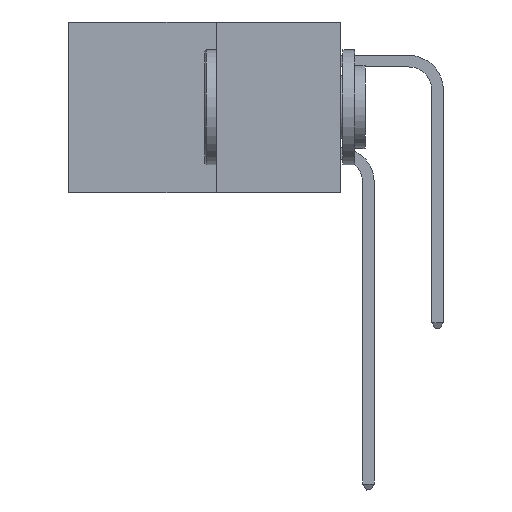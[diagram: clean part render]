
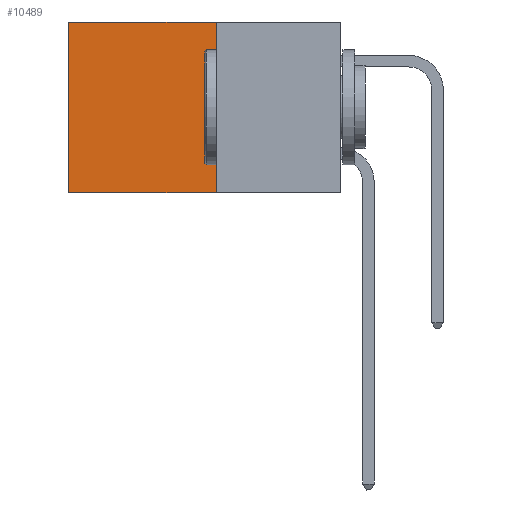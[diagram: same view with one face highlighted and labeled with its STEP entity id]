
A CAD part, left-side view. The second image highlights one B-rep face of the part: STEP entity #10489.
In plain terms, the highlighted planar face has unit normal (-1, 0, 0).
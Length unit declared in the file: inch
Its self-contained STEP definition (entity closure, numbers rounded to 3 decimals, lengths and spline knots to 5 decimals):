
#34 = DIRECTION ( 'NONE',  ( 0., 1., 0. ) ) ;
#147 = EDGE_CURVE ( 'NONE', #11478, #3069, #4063, .T. ) ;
#631 = VERTEX_POINT ( 'NONE', #3642 ) ;
#1142 = VECTOR ( 'NONE', #6625, 39.37008 ) ;
#1674 = DIRECTION ( 'NONE',  ( 0., 0., -1. ) ) ;
#1857 = CARTESIAN_POINT ( 'NONE',  ( 0.277, 0.59, -0.37 ) ) ;
#2637 = CARTESIAN_POINT ( 'NONE',  ( 0.277, 0.27, -0.37 ) ) ;
#3069 = VERTEX_POINT ( 'NONE', #1857 ) ;
#3433 = CARTESIAN_POINT ( 'NONE',  ( 0.277, 0.27, 0. ) ) ;
#3642 = CARTESIAN_POINT ( 'NONE',  ( 0.277, 0.27, 0. ) ) ;
#3897 = VERTEX_POINT ( 'NONE', #13266 ) ;
#4063 = LINE ( 'NONE', #9740, #1142 ) ;
#4316 = ORIENTED_EDGE ( 'NONE', *, *, #8515, .F. ) ;
#4491 = EDGE_LOOP ( 'NONE', ( #4612, #10449, #4316, #14086 ) ) ;
#4612 = ORIENTED_EDGE ( 'NONE', *, *, #147, .T. ) ;
#4622 = DIRECTION ( 'NONE',  ( 0., 1., 0. ) ) ;
#4642 = VECTOR ( 'NONE', #4622, 39.37008 ) ;
#4816 = FACE_OUTER_BOUND ( 'NONE', #4491, .T. ) ;
#5504 = AXIS2_PLACEMENT_3D ( 'NONE', #7200, #8316, #1674 ) ;
#5690 = EDGE_CURVE ( 'NONE', #3897, #3069, #11979, .T. ) ;
#6625 = DIRECTION ( 'NONE',  ( 0., 0., -1. ) ) ;
#6769 = LINE ( 'NONE', #2637, #9718 ) ;
#7200 = CARTESIAN_POINT ( 'NONE',  ( 0.277, 0.27, -0.37 ) ) ;
#8316 = DIRECTION ( 'NONE',  ( 1., 0., 0. ) ) ;
#8515 = EDGE_CURVE ( 'NONE', #631, #3897, #6769, .T. ) ;
#8974 = VECTOR ( 'NONE', #34, 39.37008 ) ;
#9183 = DIRECTION ( 'NONE',  ( 0., 0., -1. ) ) ;
#9718 = VECTOR ( 'NONE', #9183, 39.37008 ) ;
#9740 = CARTESIAN_POINT ( 'NONE',  ( 0.277, 0.59, -0.37 ) ) ;
#10269 = EDGE_CURVE ( 'NONE', #631, #11478, #14277, .T. ) ;
#10449 = ORIENTED_EDGE ( 'NONE', *, *, #5690, .F. ) ;
#10489 = ADVANCED_FACE ( 'NONE', ( #4816 ), #13903, .F. ) ;
#11478 = VERTEX_POINT ( 'NONE', #14312 ) ;
#11979 = LINE ( 'NONE', #13374, #8974 ) ;
#13266 = CARTESIAN_POINT ( 'NONE',  ( 0.277, 0.27, -0.37 ) ) ;
#13374 = CARTESIAN_POINT ( 'NONE',  ( 0.277, 0.27, -0.37 ) ) ;
#13903 = PLANE ( 'NONE',  #5504 ) ;
#14086 = ORIENTED_EDGE ( 'NONE', *, *, #10269, .T. ) ;
#14277 = LINE ( 'NONE', #3433, #4642 ) ;
#14312 = CARTESIAN_POINT ( 'NONE',  ( 0.277, 0.59, 0. ) ) ;
